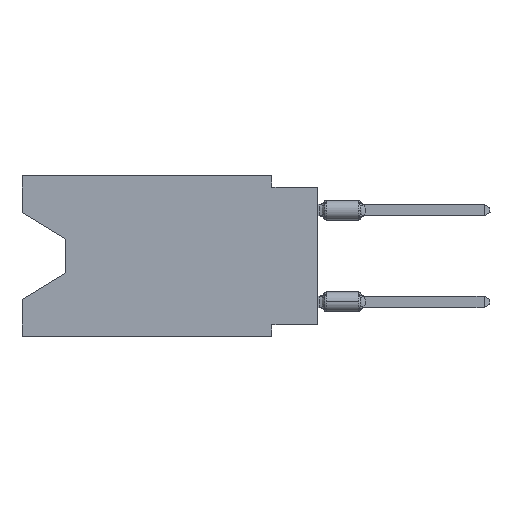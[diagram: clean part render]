
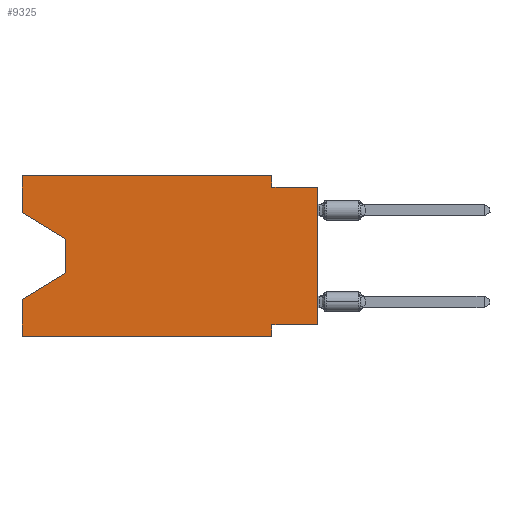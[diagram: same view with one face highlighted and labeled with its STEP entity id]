
A CAD part, left-side view. The second image highlights one B-rep face of the part: STEP entity #9325.
In plain terms, the highlighted planar face has unit normal (-1, 0, 0).
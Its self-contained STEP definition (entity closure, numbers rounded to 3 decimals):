
#145 = ORIENTED_EDGE ( 'NONE', *, *, #17553, .F. ) ;
#300 = CARTESIAN_POINT ( 'NONE',  ( 0., 0., -8.255 ) ) ;
#1033 = EDGE_CURVE ( 'NONE', #26912, #33397, #20620, .T. ) ;
#1397 = ORIENTED_EDGE ( 'NONE', *, *, #1033, .T. ) ;
#2256 = ORIENTED_EDGE ( 'NONE', *, *, #20244, .T. ) ;
#2702 = VERTEX_POINT ( 'NONE', #15802 ) ;
#2824 = VERTEX_POINT ( 'NONE', #23606 ) ;
#3010 = DIRECTION ( 'NONE',  ( 0., 0., -1. ) ) ;
#3933 = EDGE_CURVE ( 'NONE', #2824, #22492, #11900, .T. ) ;
#3937 = DIRECTION ( 'NONE',  ( 0., 0., 1. ) ) ;
#4038 = ORIENTED_EDGE ( 'NONE', *, *, #15476, .F. ) ;
#4052 = CARTESIAN_POINT ( 'NONE',  ( 0., 16.383, 0. ) ) ;
#4097 = CARTESIAN_POINT ( 'NONE',  ( 0., 16.383, 0. ) ) ;
#4366 = CARTESIAN_POINT ( 'NONE',  ( 0., 0., 0. ) ) ;
#4405 = VERTEX_POINT ( 'NONE', #26069 ) ;
#4525 = LINE ( 'NONE', #15355, #7334 ) ;
#5293 = DIRECTION ( 'NONE',  ( 0., -1., 0. ) ) ;
#6936 = CARTESIAN_POINT ( 'NONE',  ( 0., 16.383, 0. ) ) ;
#7334 = VECTOR ( 'NONE', #7353, 1000. ) ;
#7353 = DIRECTION ( 'NONE',  ( 0., -1., 0. ) ) ;
#7845 = DIRECTION ( 'NONE',  ( 0., 0., -1. ) ) ;
#8118 = LINE ( 'NONE', #300, #32776 ) ;
#8647 = LINE ( 'NONE', #11842, #23651 ) ;
#8862 = DIRECTION ( 'NONE',  ( 0., 0., -1. ) ) ;
#9325 = ADVANCED_FACE ( 'NONE', ( #19889 ), #30727, .F. ) ;
#9560 = CARTESIAN_POINT ( 'NONE',  ( 0., 13.97, -5.385 ) ) ;
#9774 = LINE ( 'NONE', #6936, #30337 ) ;
#9806 = VERTEX_POINT ( 'NONE', #12893 ) ;
#10027 = DIRECTION ( 'NONE',  ( 0., 0., 1. ) ) ;
#10103 = LINE ( 'NONE', #18977, #31748 ) ;
#10517 = LINE ( 'NONE', #21354, #30488 ) ;
#11349 = VECTOR ( 'NONE', #22742, 1000. ) ;
#11537 = EDGE_CURVE ( 'NONE', #33696, #9806, #4525, .T. ) ;
#11842 = CARTESIAN_POINT ( 'NONE',  ( 0., 16.383, -2.038 ) ) ;
#11900 = LINE ( 'NONE', #4097, #11349 ) ;
#12421 = CARTESIAN_POINT ( 'NONE',  ( 0., 16.383, 0. ) ) ;
#12600 = DIRECTION ( 'NONE',  ( 0., 0., -1. ) ) ;
#12769 = LINE ( 'NONE', #26458, #29832 ) ;
#12800 = CARTESIAN_POINT ( 'NONE',  ( 0., 13.97, -5.385 ) ) ;
#12893 = CARTESIAN_POINT ( 'NONE',  ( 0., 2.54, -8.89 ) ) ;
#14534 = VERTEX_POINT ( 'NONE', #30854 ) ;
#15134 = DIRECTION ( 'NONE',  ( 0., 0.855, -0.519 ) ) ;
#15150 = ORIENTED_EDGE ( 'NONE', *, *, #25555, .T. ) ;
#15350 = EDGE_CURVE ( 'NONE', #32423, #14534, #33758, .T. ) ;
#15355 = CARTESIAN_POINT ( 'NONE',  ( 0., 16.383, -8.89 ) ) ;
#15440 = CARTESIAN_POINT ( 'NONE',  ( 0., 2.54, -8.255 ) ) ;
#15476 = EDGE_CURVE ( 'NONE', #22492, #4405, #10103, .T. ) ;
#15802 = CARTESIAN_POINT ( 'NONE',  ( 0., 0., -8.255 ) ) ;
#16141 = DIRECTION ( 'NONE',  ( 0., 1., 0. ) ) ;
#16895 = ORIENTED_EDGE ( 'NONE', *, *, #29402, .F. ) ;
#17553 = EDGE_CURVE ( 'NONE', #4405, #32423, #12769, .T. ) ;
#17563 = VERTEX_POINT ( 'NONE', #15440 ) ;
#18977 = CARTESIAN_POINT ( 'NONE',  ( 0., 16.383, 0. ) ) ;
#19126 = VECTOR ( 'NONE', #15134, 1000. ) ;
#19889 = FACE_OUTER_BOUND ( 'NONE', #24229, .T. ) ;
#20176 = ORIENTED_EDGE ( 'NONE', *, *, #28875, .T. ) ;
#20244 = EDGE_CURVE ( 'NONE', #2824, #23017, #8647, .T. ) ;
#20420 = DIRECTION ( 'NONE',  ( 0., -1., 0. ) ) ;
#20620 = LINE ( 'NONE', #12800, #19126 ) ;
#21090 = EDGE_CURVE ( 'NONE', #2702, #17563, #8118, .T. ) ;
#21354 = CARTESIAN_POINT ( 'NONE',  ( 0., 2.54, -8.89 ) ) ;
#22492 = VERTEX_POINT ( 'NONE', #4052 ) ;
#22742 = DIRECTION ( 'NONE',  ( 0., 0., 1. ) ) ;
#23017 = VERTEX_POINT ( 'NONE', #25318 ) ;
#23232 = VECTOR ( 'NONE', #20420, 1000. ) ;
#23606 = CARTESIAN_POINT ( 'NONE',  ( 0., 16.383, -2.038 ) ) ;
#23651 = VECTOR ( 'NONE', #26833, 1000. ) ;
#23781 = CARTESIAN_POINT ( 'NONE',  ( 0., 2.54, -0.635 ) ) ;
#23841 = AXIS2_PLACEMENT_3D ( 'NONE', #12421, #33221, #8862 ) ;
#24229 = EDGE_LOOP ( 'NONE', ( #2256, #15150, #1397, #24681, #30039, #16895, #32902, #20176, #33090, #145, #4038, #27660 ) ) ;
#24681 = ORIENTED_EDGE ( 'NONE', *, *, #26557, .F. ) ;
#25318 = CARTESIAN_POINT ( 'NONE',  ( 0., 13.97, -3.505 ) ) ;
#25396 = CARTESIAN_POINT ( 'NONE',  ( 0., 0., -0.635 ) ) ;
#25555 = EDGE_CURVE ( 'NONE', #23017, #26912, #27344, .T. ) ;
#25913 = VECTOR ( 'NONE', #10027, 1000. ) ;
#26069 = CARTESIAN_POINT ( 'NONE',  ( 0., 2.54, 0. ) ) ;
#26458 = CARTESIAN_POINT ( 'NONE',  ( 0., 2.54, 0. ) ) ;
#26557 = EDGE_CURVE ( 'NONE', #33696, #33397, #9774, .T. ) ;
#26833 = DIRECTION ( 'NONE',  ( 0., -0.855, -0.519 ) ) ;
#26912 = VERTEX_POINT ( 'NONE', #9560 ) ;
#27344 = LINE ( 'NONE', #32506, #34353 ) ;
#27660 = ORIENTED_EDGE ( 'NONE', *, *, #3933, .F. ) ;
#28691 = LINE ( 'NONE', #4366, #25913 ) ;
#28875 = EDGE_CURVE ( 'NONE', #2702, #14534, #28691, .T. ) ;
#29402 = EDGE_CURVE ( 'NONE', #17563, #9806, #10517, .T. ) ;
#29555 = CARTESIAN_POINT ( 'NONE',  ( 0., 16.383, -6.852 ) ) ;
#29832 = VECTOR ( 'NONE', #12600, 1000. ) ;
#30039 = ORIENTED_EDGE ( 'NONE', *, *, #11537, .T. ) ;
#30337 = VECTOR ( 'NONE', #3937, 1000. ) ;
#30488 = VECTOR ( 'NONE', #7845, 1000. ) ;
#30727 = PLANE ( 'NONE',  #23841 ) ;
#30854 = CARTESIAN_POINT ( 'NONE',  ( 0., 0., -0.635 ) ) ;
#31748 = VECTOR ( 'NONE', #5293, 1000. ) ;
#32423 = VERTEX_POINT ( 'NONE', #23781 ) ;
#32506 = CARTESIAN_POINT ( 'NONE',  ( 0., 13.97, -3.505 ) ) ;
#32776 = VECTOR ( 'NONE', #16141, 1000. ) ;
#32902 = ORIENTED_EDGE ( 'NONE', *, *, #21090, .F. ) ;
#33023 = CARTESIAN_POINT ( 'NONE',  ( 0., 16.383, -8.89 ) ) ;
#33090 = ORIENTED_EDGE ( 'NONE', *, *, #15350, .F. ) ;
#33221 = DIRECTION ( 'NONE',  ( 1., 0., 0. ) ) ;
#33397 = VERTEX_POINT ( 'NONE', #29555 ) ;
#33696 = VERTEX_POINT ( 'NONE', #33023 ) ;
#33758 = LINE ( 'NONE', #25396, #23232 ) ;
#34353 = VECTOR ( 'NONE', #3010, 1000. ) ;
